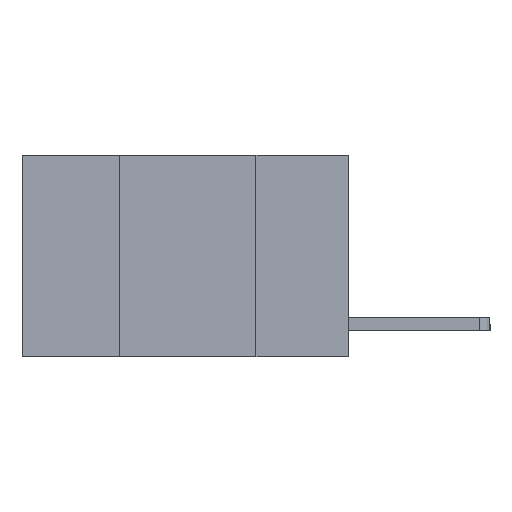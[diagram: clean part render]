
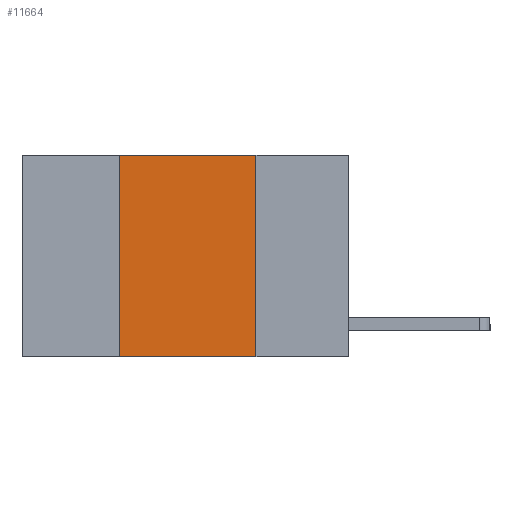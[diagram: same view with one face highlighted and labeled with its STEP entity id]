
A CAD part, left-side view. The second image highlights one B-rep face of the part: STEP entity #11664.
In plain terms, the highlighted planar face has unit normal (-1, 0, 0).
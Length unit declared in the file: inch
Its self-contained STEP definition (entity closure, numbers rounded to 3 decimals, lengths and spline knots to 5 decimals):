
#44 = EDGE_CURVE ( 'NONE', #9803, #124, #7359, .T. ) ;
#124 = VERTEX_POINT ( 'NONE', #8129 ) ;
#1829 = CARTESIAN_POINT ( 'NONE',  ( 0., 0.6, -0.37 ) ) ;
#2436 = CARTESIAN_POINT ( 'NONE',  ( 0., 0.42, 0. ) ) ;
#2625 = ORIENTED_EDGE ( 'NONE', *, *, #4816, .F. ) ;
#2639 = VECTOR ( 'NONE', #6405, 39.37008 ) ;
#2991 = LINE ( 'NONE', #4878, #9408 ) ;
#3100 = DIRECTION ( 'NONE',  ( 0., 0., 1. ) ) ;
#3619 = VECTOR ( 'NONE', #11608, 39.37008 ) ;
#4336 = CARTESIAN_POINT ( 'NONE',  ( 0., 0.17, 0. ) ) ;
#4675 = EDGE_CURVE ( 'NONE', #9803, #6425, #7854, .T. ) ;
#4816 = EDGE_CURVE ( 'NONE', #11236, #124, #9754, .T. ) ;
#4878 = CARTESIAN_POINT ( 'NONE',  ( 0., 0.6, 0. ) ) ;
#5006 = DIRECTION ( 'NONE',  ( 1., 0., 0. ) ) ;
#6168 = ORIENTED_EDGE ( 'NONE', *, *, #44, .T. ) ;
#6272 = VECTOR ( 'NONE', #3100, 39.37008 ) ;
#6370 = AXIS2_PLACEMENT_3D ( 'NONE', #9649, #5006, #8640 ) ;
#6405 = DIRECTION ( 'NONE',  ( 0., -1., 0. ) ) ;
#6425 = VERTEX_POINT ( 'NONE', #6800 ) ;
#6800 = CARTESIAN_POINT ( 'NONE',  ( 0., 0.42, 0. ) ) ;
#7359 = LINE ( 'NONE', #1829, #2639 ) ;
#7611 = ORIENTED_EDGE ( 'NONE', *, *, #4675, .F. ) ;
#7820 = CARTESIAN_POINT ( 'NONE',  ( 0., 0.42, -0.37 ) ) ;
#7854 = LINE ( 'NONE', #2436, #6272 ) ;
#7997 = CARTESIAN_POINT ( 'NONE',  ( 0., 0.17, 0. ) ) ;
#8129 = CARTESIAN_POINT ( 'NONE',  ( 0., 0.17, -0.37 ) ) ;
#8640 = DIRECTION ( 'NONE',  ( 0., 0., -1. ) ) ;
#9408 = VECTOR ( 'NONE', #11204, 39.37008 ) ;
#9592 = PLANE ( 'NONE',  #6370 ) ;
#9649 = CARTESIAN_POINT ( 'NONE',  ( 0., 0.6, 0. ) ) ;
#9754 = LINE ( 'NONE', #4336, #3619 ) ;
#9803 = VERTEX_POINT ( 'NONE', #7820 ) ;
#10426 = FACE_OUTER_BOUND ( 'NONE', #11084, .T. ) ;
#11084 = EDGE_LOOP ( 'NONE', ( #2625, #11182, #7611, #6168 ) ) ;
#11182 = ORIENTED_EDGE ( 'NONE', *, *, #11373, .F. ) ;
#11204 = DIRECTION ( 'NONE',  ( 0., -1., 0. ) ) ;
#11236 = VERTEX_POINT ( 'NONE', #7997 ) ;
#11373 = EDGE_CURVE ( 'NONE', #6425, #11236, #2991, .T. ) ;
#11608 = DIRECTION ( 'NONE',  ( 0., 0., -1. ) ) ;
#11664 = ADVANCED_FACE ( 'NONE', ( #10426 ), #9592, .F. ) ;
